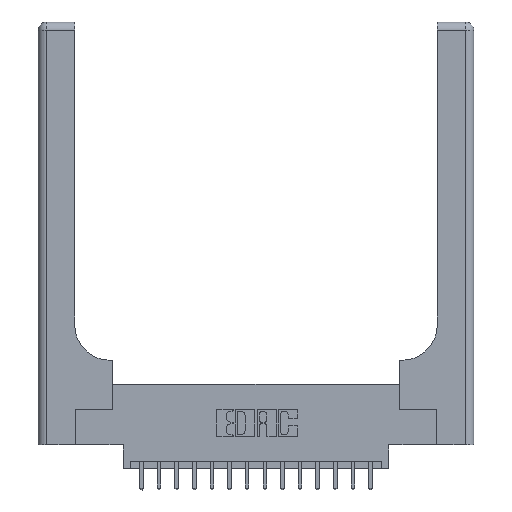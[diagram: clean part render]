
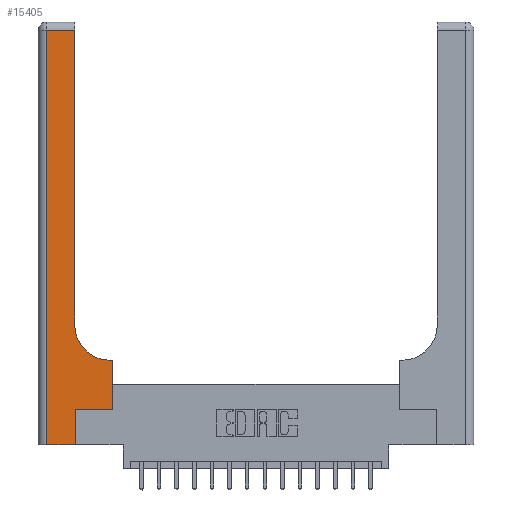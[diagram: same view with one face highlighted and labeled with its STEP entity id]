
A CAD part, top view. The second image highlights one B-rep face of the part: STEP entity #15405.
In plain terms, the highlighted planar face has unit normal (0, 0, 1).
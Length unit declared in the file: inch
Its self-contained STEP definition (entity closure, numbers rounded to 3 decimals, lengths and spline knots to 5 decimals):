
#33 = EDGE_CURVE ( 'NONE', #13996, #10426, #4166, .T. ) ;
#1083 = DIRECTION ( 'NONE',  ( 0., -1., 0. ) ) ;
#1097 = ORIENTED_EDGE ( 'NONE', *, *, #7673, .T. ) ;
#1273 = DIRECTION ( 'NONE',  ( 1., 0., 0. ) ) ;
#1536 = CARTESIAN_POINT ( 'NONE',  ( 0., 0., 0.37 ) ) ;
#1613 = VERTEX_POINT ( 'NONE', #9717 ) ;
#1800 = DIRECTION ( 'NONE',  ( 1., 0., 0. ) ) ;
#2592 = VERTEX_POINT ( 'NONE', #12288 ) ;
#2923 = VECTOR ( 'NONE', #1083, 39.37008 ) ;
#3163 = FACE_OUTER_BOUND ( 'NONE', #6032, .T. ) ;
#3221 = CARTESIAN_POINT ( 'NONE',  ( 0.265, 0.25, 0.37 ) ) ;
#3575 = DIRECTION ( 'NONE',  ( -1., 0., 0. ) ) ;
#3584 = VECTOR ( 'NONE', #11202, 39.37008 ) ;
#3713 = VECTOR ( 'NONE', #4733, 39.37008 ) ;
#4049 = LINE ( 'NONE', #6925, #3584 ) ;
#4166 = LINE ( 'NONE', #16585, #3713 ) ;
#4391 = DIRECTION ( 'NONE',  ( 1., 0., 0. ) ) ;
#4733 = DIRECTION ( 'NONE',  ( 0., 1., 0. ) ) ;
#5052 = DIRECTION ( 'NONE',  ( 0., 1., 0. ) ) ;
#5566 = CARTESIAN_POINT ( 'NONE',  ( 0.528, 0.6, 0.37 ) ) ;
#5651 = VERTEX_POINT ( 'NONE', #11531 ) ;
#5736 = ORIENTED_EDGE ( 'NONE', *, *, #18053, .T. ) ;
#5755 = EDGE_CURVE ( 'NONE', #10426, #10712, #5771, .T. ) ;
#5771 = LINE ( 'NONE', #3221, #12851 ) ;
#6032 = EDGE_LOOP ( 'NONE', ( #7131, #15202, #15045, #1097, #17392, #17093, #12034, #16606, #5736 ) ) ;
#6088 = LINE ( 'NONE', #1536, #13162 ) ;
#6392 = LINE ( 'NONE', #17622, #13469 ) ;
#6499 = DIRECTION ( 'NONE',  ( -1., 0., 0. ) ) ;
#6696 = LINE ( 'NONE', #16567, #2923 ) ;
#6925 = CARTESIAN_POINT ( 'NONE',  ( 0.528, 0.25, 0.37 ) ) ;
#7077 = CARTESIAN_POINT ( 'NONE',  ( 0.265, 0., 0.37 ) ) ;
#7131 = ORIENTED_EDGE ( 'NONE', *, *, #12147, .T. ) ;
#7673 = EDGE_CURVE ( 'NONE', #2592, #13996, #6088, .T. ) ;
#7842 = AXIS2_PLACEMENT_3D ( 'NONE', #16180, #12047, #3575 ) ;
#8440 = CARTESIAN_POINT ( 'NONE',  ( 0.26, 2.94, 0.37 ) ) ;
#8740 = DIRECTION ( 'NONE',  ( -1., 0., 0. ) ) ;
#8752 = LINE ( 'NONE', #14953, #12521 ) ;
#9717 = CARTESIAN_POINT ( 'NONE',  ( 0.51, 0.6, 0.37 ) ) ;
#9760 = DIRECTION ( 'NONE',  ( 0., 0., -1. ) ) ;
#10195 = EDGE_CURVE ( 'NONE', #10712, #15632, #4049, .T. ) ;
#10260 = CARTESIAN_POINT ( 'NONE',  ( 0.265, 0.25, 0.37 ) ) ;
#10426 = VERTEX_POINT ( 'NONE', #10260 ) ;
#10613 = PLANE ( 'NONE',  #7842 ) ;
#10666 = VERTEX_POINT ( 'NONE', #15057 ) ;
#10712 = VERTEX_POINT ( 'NONE', #15107 ) ;
#11202 = DIRECTION ( 'NONE',  ( 0., 1., 0. ) ) ;
#11531 = CARTESIAN_POINT ( 'NONE',  ( 0.06, 2.94, 0.37 ) ) ;
#12034 = ORIENTED_EDGE ( 'NONE', *, *, #10195, .T. ) ;
#12047 = DIRECTION ( 'NONE',  ( 0., 0., -1. ) ) ;
#12147 = EDGE_CURVE ( 'NONE', #10666, #16238, #6392, .T. ) ;
#12288 = CARTESIAN_POINT ( 'NONE',  ( 0.06, 0., 0.37 ) ) ;
#12521 = VECTOR ( 'NONE', #6499, 39.37008 ) ;
#12851 = VECTOR ( 'NONE', #1800, 39.37008 ) ;
#12954 = CARTESIAN_POINT ( 'NONE',  ( 0., 2.94, 0.37 ) ) ;
#13162 = VECTOR ( 'NONE', #4391, 39.37008 ) ;
#13337 = VECTOR ( 'NONE', #8740, 39.37008 ) ;
#13469 = VECTOR ( 'NONE', #5052, 39.37008 ) ;
#13996 = VERTEX_POINT ( 'NONE', #7077 ) ;
#14353 = EDGE_CURVE ( 'NONE', #15632, #1613, #8752, .T. ) ;
#14406 = CIRCLE ( 'NONE', #14830, 0.25 ) ;
#14830 = AXIS2_PLACEMENT_3D ( 'NONE', #18123, #9760, #1273 ) ;
#14953 = CARTESIAN_POINT ( 'NONE',  ( 0.26, 0.6, 0.37 ) ) ;
#15045 = ORIENTED_EDGE ( 'NONE', *, *, #16830, .T. ) ;
#15057 = CARTESIAN_POINT ( 'NONE',  ( 0.26, 0.85, 0.37 ) ) ;
#15107 = CARTESIAN_POINT ( 'NONE',  ( 0.528, 0.25, 0.37 ) ) ;
#15202 = ORIENTED_EDGE ( 'NONE', *, *, #16383, .T. ) ;
#15405 = ADVANCED_FACE ( 'NONE', ( #3163 ), #10613, .F. ) ;
#15632 = VERTEX_POINT ( 'NONE', #5566 ) ;
#16180 = CARTESIAN_POINT ( 'NONE',  ( 0., 3., 0.37 ) ) ;
#16238 = VERTEX_POINT ( 'NONE', #8440 ) ;
#16383 = EDGE_CURVE ( 'NONE', #16238, #5651, #17038, .T. ) ;
#16567 = CARTESIAN_POINT ( 'NONE',  ( 0.06, 3., 0.37 ) ) ;
#16585 = CARTESIAN_POINT ( 'NONE',  ( 0.265, 0., 0.37 ) ) ;
#16606 = ORIENTED_EDGE ( 'NONE', *, *, #14353, .T. ) ;
#16830 = EDGE_CURVE ( 'NONE', #5651, #2592, #6696, .T. ) ;
#17038 = LINE ( 'NONE', #12954, #13337 ) ;
#17093 = ORIENTED_EDGE ( 'NONE', *, *, #5755, .T. ) ;
#17392 = ORIENTED_EDGE ( 'NONE', *, *, #33, .T. ) ;
#17622 = CARTESIAN_POINT ( 'NONE',  ( 0.26, 3., 0.37 ) ) ;
#18053 = EDGE_CURVE ( 'NONE', #1613, #10666, #14406, .T. ) ;
#18123 = CARTESIAN_POINT ( 'NONE',  ( 0.51, 0.85, 0.37 ) ) ;
